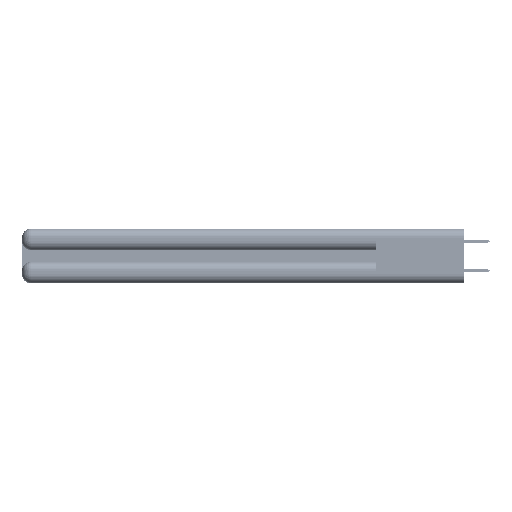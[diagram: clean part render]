
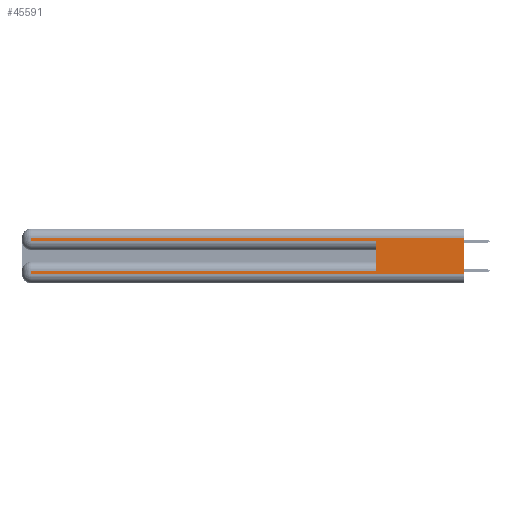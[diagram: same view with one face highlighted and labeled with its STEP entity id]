
A CAD part, left-side view. The second image highlights one B-rep face of the part: STEP entity #45591.
In plain terms, the highlighted planar face has unit normal (-1, 0, 0).
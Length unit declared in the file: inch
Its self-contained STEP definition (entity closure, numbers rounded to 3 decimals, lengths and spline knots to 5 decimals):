
#618 = CARTESIAN_POINT ( 'NONE',  ( 0., 0., 0.06 ) ) ;
#4284 = VERTEX_POINT ( 'NONE', #618 ) ;
#4430 = CARTESIAN_POINT ( 'NONE',  ( 0., 2.94, 0.37 ) ) ;
#4475 = LINE ( 'NONE', #28016, #12891 ) ;
#4749 = EDGE_CURVE ( 'NONE', #22386, #4284, #39496, .T. ) ;
#5351 = VERTEX_POINT ( 'NONE', #24326 ) ;
#5681 = ORIENTED_EDGE ( 'NONE', *, *, #11821, .T. ) ;
#6969 = CARTESIAN_POINT ( 'NONE',  ( 0., 0.6, 0.145 ) ) ;
#7425 = ORIENTED_EDGE ( 'NONE', *, *, #29426, .T. ) ;
#7591 = DIRECTION ( 'NONE',  ( 0., 0., -1. ) ) ;
#9547 = DIRECTION ( 'NONE',  ( 0., -1., 0. ) ) ;
#11272 = CARTESIAN_POINT ( 'NONE',  ( 0., 0., 0.31 ) ) ;
#11821 = EDGE_CURVE ( 'NONE', #56902, #5351, #18390, .T. ) ;
#12329 = CARTESIAN_POINT ( 'NONE',  ( 0., 0., 0.285 ) ) ;
#12891 = VECTOR ( 'NONE', #50003, 39.37008 ) ;
#13631 = DIRECTION ( 'NONE',  ( 0., 0., -1. ) ) ;
#16168 = DIRECTION ( 'NONE',  ( 0., 0., 1. ) ) ;
#16197 = CARTESIAN_POINT ( 'NONE',  ( 0., 0., 0.37 ) ) ;
#16464 = PLANE ( 'NONE',  #54182 ) ;
#17724 = VECTOR ( 'NONE', #55562, 39.37008 ) ;
#18390 = LINE ( 'NONE', #51280, #17724 ) ;
#18649 = VERTEX_POINT ( 'NONE', #36064 ) ;
#20890 = ORIENTED_EDGE ( 'NONE', *, *, #47904, .T. ) ;
#21380 = CARTESIAN_POINT ( 'NONE',  ( 0., 0., 0.37 ) ) ;
#21898 = CARTESIAN_POINT ( 'NONE',  ( 0., 2.94, 0.31 ) ) ;
#22386 = VERTEX_POINT ( 'NONE', #27788 ) ;
#24326 = CARTESIAN_POINT ( 'NONE',  ( 0., 2.94, 0.085 ) ) ;
#24722 = LINE ( 'NONE', #16197, #42817 ) ;
#25406 = EDGE_CURVE ( 'NONE', #33413, #4284, #24722, .T. ) ;
#25585 = VERTEX_POINT ( 'NONE', #21898 ) ;
#25659 = EDGE_LOOP ( 'NONE', ( #37648, #20890, #27780, #7425, #28257, #5681, #35102, #37776 ) ) ;
#25662 = EDGE_CURVE ( 'NONE', #5351, #22386, #32400, .T. ) ;
#25861 = DIRECTION ( 'NONE',  ( 1., 0., 0. ) ) ;
#26609 = DIRECTION ( 'NONE',  ( 0., -1., 0. ) ) ;
#26959 = VECTOR ( 'NONE', #9547, 39.37008 ) ;
#27007 = VECTOR ( 'NONE', #26609, 39.37008 ) ;
#27780 = ORIENTED_EDGE ( 'NONE', *, *, #57686, .T. ) ;
#27788 = CARTESIAN_POINT ( 'NONE',  ( 0., 2.94, 0.06 ) ) ;
#28016 = CARTESIAN_POINT ( 'NONE',  ( 0., 2.94, 0.37 ) ) ;
#28257 = ORIENTED_EDGE ( 'NONE', *, *, #55254, .F. ) ;
#28927 = CARTESIAN_POINT ( 'NONE',  ( 0., 0., 0.31 ) ) ;
#29426 = EDGE_CURVE ( 'NONE', #36800, #18649, #29807, .T. ) ;
#29807 = LINE ( 'NONE', #12329, #27007 ) ;
#30359 = DIRECTION ( 'NONE',  ( 0., 0., -1. ) ) ;
#31003 = VECTOR ( 'NONE', #13631, 39.37008 ) ;
#32400 = LINE ( 'NONE', #4430, #31003 ) ;
#33413 = VERTEX_POINT ( 'NONE', #11272 ) ;
#33657 = CARTESIAN_POINT ( 'NONE',  ( 0., 2.94, 0.285 ) ) ;
#35102 = ORIENTED_EDGE ( 'NONE', *, *, #25662, .T. ) ;
#36064 = CARTESIAN_POINT ( 'NONE',  ( 0., 0.6, 0.285 ) ) ;
#36800 = VERTEX_POINT ( 'NONE', #33657 ) ;
#37648 = ORIENTED_EDGE ( 'NONE', *, *, #25406, .F. ) ;
#37776 = ORIENTED_EDGE ( 'NONE', *, *, #4749, .T. ) ;
#39496 = LINE ( 'NONE', #40235, #26959 ) ;
#40235 = CARTESIAN_POINT ( 'NONE',  ( 0., 0., 0.06 ) ) ;
#42817 = VECTOR ( 'NONE', #7591, 39.37008 ) ;
#42935 = FACE_OUTER_BOUND ( 'NONE', #25659, .T. ) ;
#44277 = VECTOR ( 'NONE', #16168, 39.37008 ) ;
#45510 = VECTOR ( 'NONE', #51107, 39.37008 ) ;
#45591 = ADVANCED_FACE ( 'NONE', ( #42935 ), #16464, .F. ) ;
#47904 = EDGE_CURVE ( 'NONE', #33413, #25585, #52470, .T. ) ;
#50003 = DIRECTION ( 'NONE',  ( 0., 0., -1. ) ) ;
#51107 = DIRECTION ( 'NONE',  ( 0., 1., 0. ) ) ;
#51280 = CARTESIAN_POINT ( 'NONE',  ( 0., 0., 0.085 ) ) ;
#52470 = LINE ( 'NONE', #28927, #45510 ) ;
#52695 = CARTESIAN_POINT ( 'NONE',  ( 0., 0.6, 0.085 ) ) ;
#54182 = AXIS2_PLACEMENT_3D ( 'NONE', #21380, #25861, #30359 ) ;
#55254 = EDGE_CURVE ( 'NONE', #56902, #18649, #56102, .T. ) ;
#55562 = DIRECTION ( 'NONE',  ( 0., 1., 0. ) ) ;
#56102 = LINE ( 'NONE', #6969, #44277 ) ;
#56902 = VERTEX_POINT ( 'NONE', #52695 ) ;
#57686 = EDGE_CURVE ( 'NONE', #25585, #36800, #4475, .T. ) ;
